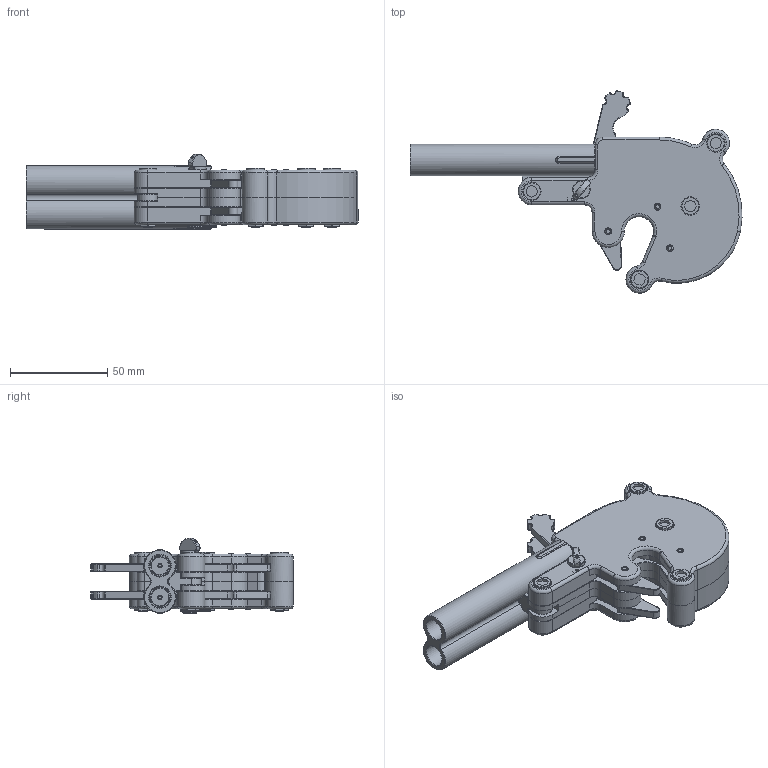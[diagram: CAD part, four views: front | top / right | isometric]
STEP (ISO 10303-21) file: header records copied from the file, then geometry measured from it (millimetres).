
FILE_DESCRIPTION(/* description */ (''),/* implementation_level */ '2;1');
FILE_NAME(/* name */ 'Derringer.stp',/* time_stamp */ '2013-08-01T09:26:30-03:00',/* author */ ('PNL'),/* organization */ (''),/* preprocessor_version */ 'ST-DEVELOPER v15.2',/* originating_system */ 'Autodesk Inventor 2014',/* authorisation */ '');
FILE_SCHEMA (('AUTOMOTIVE_DESIGN { 1 0 10303 214 3 1 1 }'));
Length unit declared in the file: millimetre
Products named in the file (21): Frame-L; Barrel; hammer; spring; trigger; Grip-L; Frame-R; Grip-R; Lock-Pin-Washer; Lock-Pin; Barrel-Bolt; Main-Spring-Bended-Spring; Barrel-Nut; Barrel-SS-Insert; Extractor-Body; Pellets-Ring; Pellets-Case; Pellets-Paper; Pellets-Cartridge; 22LR-Shell; Derringer
Bounding box: 170.47 x 103.84 x 38.53 mm (x, y, z)
Volume: 155504.6 mm3; surface area: 98012 mm2
Topology: 158 solids, 158 shells, 2111 faces, 4843 edges, 2846 vertices
Faces by surface type: cylinder 772, torus 520, plane 430, sphere 284, bspline 103, cone 2
Full cylindrical faces by diameter (mm): 2 x2, 2.95 x1, 3 x14, 3.05 x1, 3.2 x6, 3.75 x4, 4.5 x4, 5 x17, 5.58 x2, 5.74 x2, 5.77 x2, 5.86 x2, 7 x14, 7.2 x8, 7.32 x2, 9 x12, 9.175 x2, 11 x4, 11.175 x2, 11.2 x2
Entity records: 41723 total; most frequent: CARTESIAN_POINT 11279, DIRECTION 6889, ORIENTED_EDGE 5662, AXIS2_PLACEMENT_3D 2942, EDGE_CURVE 2831, VERTEX_POINT 1761, EDGE_LOOP 1604, CIRCLE 1590
